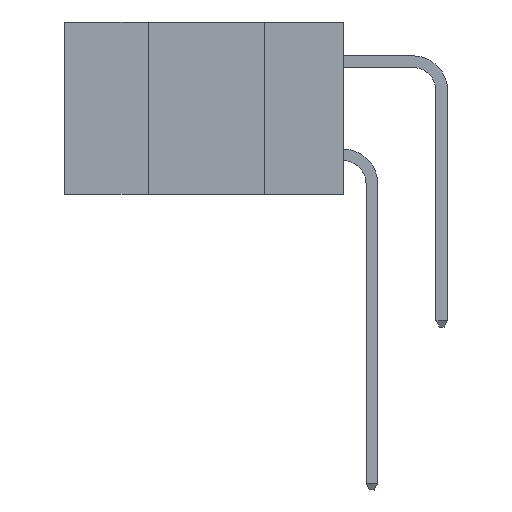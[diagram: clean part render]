
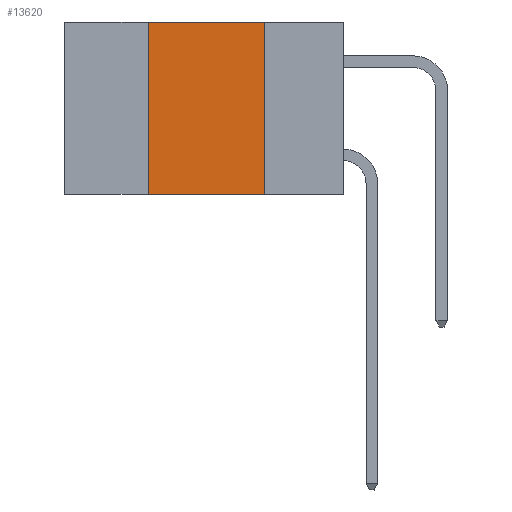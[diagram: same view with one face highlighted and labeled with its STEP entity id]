
A CAD part, left-side view. The second image highlights one B-rep face of the part: STEP entity #13620.
In plain terms, the highlighted planar face has unit normal (-1, 0, 0).
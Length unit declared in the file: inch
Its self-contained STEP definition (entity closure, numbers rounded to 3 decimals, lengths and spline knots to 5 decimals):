
#702 = EDGE_CURVE ( 'NONE', #3399, #7966, #3190, .T. ) ;
#723 = EDGE_LOOP ( 'NONE', ( #5672, #3063, #2689, #5843 ) ) ;
#928 = LINE ( 'NONE', #5314, #6975 ) ;
#1372 = VERTEX_POINT ( 'NONE', #13962 ) ;
#1557 = VECTOR ( 'NONE', #3955, 39.37008 ) ;
#1826 = AXIS2_PLACEMENT_3D ( 'NONE', #11304, #11350, #13688 ) ;
#1851 = VECTOR ( 'NONE', #3859, 39.37008 ) ;
#2107 = DIRECTION ( 'NONE',  ( 0., -1., 0. ) ) ;
#2268 = LINE ( 'NONE', #5070, #10615 ) ;
#2689 = ORIENTED_EDGE ( 'NONE', *, *, #702, .F. ) ;
#2920 = CARTESIAN_POINT ( 'NONE',  ( 0., 0.17, 0. ) ) ;
#3063 = ORIENTED_EDGE ( 'NONE', *, *, #11353, .F. ) ;
#3190 = LINE ( 'NONE', #10877, #1557 ) ;
#3399 = VERTEX_POINT ( 'NONE', #13986 ) ;
#3859 = DIRECTION ( 'NONE',  ( 0., -1., 0. ) ) ;
#3955 = DIRECTION ( 'NONE',  ( 0., 0., 1. ) ) ;
#4957 = EDGE_CURVE ( 'NONE', #3399, #1372, #14540, .T. ) ;
#5070 = CARTESIAN_POINT ( 'NONE',  ( 0., 0.17, 0. ) ) ;
#5314 = CARTESIAN_POINT ( 'NONE',  ( 0., 0.6, 0. ) ) ;
#5672 = ORIENTED_EDGE ( 'NONE', *, *, #8309, .F. ) ;
#5843 = ORIENTED_EDGE ( 'NONE', *, *, #4957, .T. ) ;
#6463 = CARTESIAN_POINT ( 'NONE',  ( 0., 0.42, 0. ) ) ;
#6975 = VECTOR ( 'NONE', #2107, 39.37008 ) ;
#7319 = CARTESIAN_POINT ( 'NONE',  ( 0., 0.6, -0.37 ) ) ;
#7966 = VERTEX_POINT ( 'NONE', #6463 ) ;
#8031 = PLANE ( 'NONE',  #1826 ) ;
#8309 = EDGE_CURVE ( 'NONE', #12291, #1372, #2268, .T. ) ;
#10615 = VECTOR ( 'NONE', #12978, 39.37008 ) ;
#10877 = CARTESIAN_POINT ( 'NONE',  ( 0., 0.42, 0. ) ) ;
#11304 = CARTESIAN_POINT ( 'NONE',  ( 0., 0.6, 0. ) ) ;
#11350 = DIRECTION ( 'NONE',  ( 1., 0., 0. ) ) ;
#11353 = EDGE_CURVE ( 'NONE', #7966, #12291, #928, .T. ) ;
#11752 = FACE_OUTER_BOUND ( 'NONE', #723, .T. ) ;
#12291 = VERTEX_POINT ( 'NONE', #2920 ) ;
#12978 = DIRECTION ( 'NONE',  ( 0., 0., -1. ) ) ;
#13620 = ADVANCED_FACE ( 'NONE', ( #11752 ), #8031, .F. ) ;
#13688 = DIRECTION ( 'NONE',  ( 0., 0., -1. ) ) ;
#13962 = CARTESIAN_POINT ( 'NONE',  ( 0., 0.17, -0.37 ) ) ;
#13986 = CARTESIAN_POINT ( 'NONE',  ( 0., 0.42, -0.37 ) ) ;
#14540 = LINE ( 'NONE', #7319, #1851 ) ;
